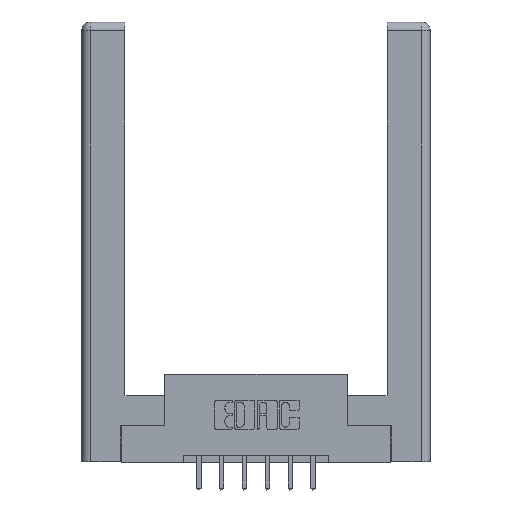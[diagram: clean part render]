
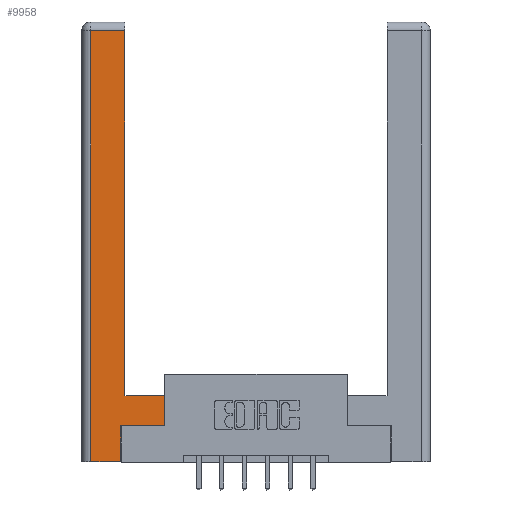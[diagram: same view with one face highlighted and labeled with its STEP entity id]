
A CAD part, top view. The second image highlights one B-rep face of the part: STEP entity #9958.
In plain terms, the highlighted planar face has unit normal (0, 0, 1).
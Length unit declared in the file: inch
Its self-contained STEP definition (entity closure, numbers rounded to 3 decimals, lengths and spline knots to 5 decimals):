
#147 = DIRECTION ( 'NONE',  ( -1., 0., 0. ) ) ;
#151 = ORIENTED_EDGE ( 'NONE', *, *, #1602, .T. ) ;
#175 = DIRECTION ( 'NONE',  ( 0., 1., 0. ) ) ;
#335 = CARTESIAN_POINT ( 'NONE',  ( 0.295, 0.45, 0. ) ) ;
#635 = CARTESIAN_POINT ( 'NONE',  ( 0.295, 2.94, 0. ) ) ;
#1460 = VECTOR ( 'NONE', #175, 39.37008 ) ;
#1470 = CARTESIAN_POINT ( 'NONE',  ( 0.565, 0.45, 0. ) ) ;
#1513 = CARTESIAN_POINT ( 'NONE',  ( 0.0615, 0., 0. ) ) ;
#1544 = VECTOR ( 'NONE', #8016, 39.37008 ) ;
#1602 = EDGE_CURVE ( 'NONE', #4958, #4509, #4754, .T. ) ;
#1690 = ORIENTED_EDGE ( 'NONE', *, *, #8846, .T. ) ;
#1697 = VECTOR ( 'NONE', #11351, 39.37008 ) ;
#1726 = LINE ( 'NONE', #1470, #5776 ) ;
#1737 = EDGE_CURVE ( 'NONE', #10759, #4958, #9622, .T. ) ;
#2299 = VECTOR ( 'NONE', #7509, 39.37008 ) ;
#2758 = VERTEX_POINT ( 'NONE', #9041 ) ;
#2831 = VECTOR ( 'NONE', #10468, 39.37008 ) ;
#3073 = VERTEX_POINT ( 'NONE', #9050 ) ;
#3211 = EDGE_LOOP ( 'NONE', ( #3826, #151, #6633, #1690, #8529, #4054, #4448, #8584 ) ) ;
#3506 = DIRECTION ( 'NONE',  ( 0., 1., 0. ) ) ;
#3643 = CARTESIAN_POINT ( 'NONE',  ( 0.0615, 0., 0. ) ) ;
#3826 = ORIENTED_EDGE ( 'NONE', *, *, #1737, .T. ) ;
#3827 = CARTESIAN_POINT ( 'NONE',  ( 0.0615, 2.94, 0. ) ) ;
#4054 = ORIENTED_EDGE ( 'NONE', *, *, #5088, .T. ) ;
#4255 = EDGE_CURVE ( 'NONE', #9108, #3073, #1726, .T. ) ;
#4448 = ORIENTED_EDGE ( 'NONE', *, *, #4255, .T. ) ;
#4509 = VERTEX_POINT ( 'NONE', #4543 ) ;
#4543 = CARTESIAN_POINT ( 'NONE',  ( 0.0615, 2.94, 0. ) ) ;
#4549 = CARTESIAN_POINT ( 'NONE',  ( 0.265, 0.245, 0. ) ) ;
#4693 = DIRECTION ( 'NONE',  ( 0., 0., -1. ) ) ;
#4754 = LINE ( 'NONE', #3827, #2299 ) ;
#4848 = FACE_OUTER_BOUND ( 'NONE', #3211, .T. ) ;
#4958 = VERTEX_POINT ( 'NONE', #635 ) ;
#5088 = EDGE_CURVE ( 'NONE', #5281, #9108, #8561, .T. ) ;
#5151 = VECTOR ( 'NONE', #8184, 39.37008 ) ;
#5281 = VERTEX_POINT ( 'NONE', #7775 ) ;
#5704 = CARTESIAN_POINT ( 'NONE',  ( 0., 0., 0. ) ) ;
#5728 = CARTESIAN_POINT ( 'NONE',  ( 0.295, 3., 0. ) ) ;
#5776 = VECTOR ( 'NONE', #3506, 39.37008 ) ;
#6212 = VECTOR ( 'NONE', #11105, 39.37008 ) ;
#6410 = CARTESIAN_POINT ( 'NONE',  ( 0.565, 0.245, 0. ) ) ;
#6633 = ORIENTED_EDGE ( 'NONE', *, *, #6708, .T. ) ;
#6708 = EDGE_CURVE ( 'NONE', #4509, #8497, #6783, .T. ) ;
#6783 = LINE ( 'NONE', #1513, #1544 ) ;
#6902 = LINE ( 'NONE', #335, #2831 ) ;
#7509 = DIRECTION ( 'NONE',  ( -1., 0., 0. ) ) ;
#7775 = CARTESIAN_POINT ( 'NONE',  ( 0.265, 0.245, 0. ) ) ;
#7872 = EDGE_CURVE ( 'NONE', #3073, #10759, #6902, .T. ) ;
#8016 = DIRECTION ( 'NONE',  ( 0., -1., 0. ) ) ;
#8184 = DIRECTION ( 'NONE',  ( 0., 1., 0. ) ) ;
#8497 = VERTEX_POINT ( 'NONE', #3643 ) ;
#8511 = CARTESIAN_POINT ( 'NONE',  ( 0.265, 0., 0. ) ) ;
#8529 = ORIENTED_EDGE ( 'NONE', *, *, #9444, .T. ) ;
#8561 = LINE ( 'NONE', #6410, #6212 ) ;
#8584 = ORIENTED_EDGE ( 'NONE', *, *, #7872, .T. ) ;
#8846 = EDGE_CURVE ( 'NONE', #8497, #2758, #12041, .T. ) ;
#9041 = CARTESIAN_POINT ( 'NONE',  ( 0.265, 0., 0. ) ) ;
#9050 = CARTESIAN_POINT ( 'NONE',  ( 0.565, 0.45, 0. ) ) ;
#9108 = VERTEX_POINT ( 'NONE', #9927 ) ;
#9444 = EDGE_CURVE ( 'NONE', #2758, #5281, #10391, .T. ) ;
#9622 = LINE ( 'NONE', #5728, #1460 ) ;
#9725 = CARTESIAN_POINT ( 'NONE',  ( 0.295, 0.45, 0. ) ) ;
#9927 = CARTESIAN_POINT ( 'NONE',  ( 0.565, 0.245, 0. ) ) ;
#9958 = ADVANCED_FACE ( 'NONE', ( #4848 ), #11304, .F. ) ;
#10391 = LINE ( 'NONE', #4549, #5151 ) ;
#10468 = DIRECTION ( 'NONE',  ( -1., 0., 0. ) ) ;
#10759 = VERTEX_POINT ( 'NONE', #9725 ) ;
#11057 = AXIS2_PLACEMENT_3D ( 'NONE', #5704, #4693, #147 ) ;
#11105 = DIRECTION ( 'NONE',  ( 1., 0., 0. ) ) ;
#11304 = PLANE ( 'NONE',  #11057 ) ;
#11351 = DIRECTION ( 'NONE',  ( 1., 0., 0. ) ) ;
#12041 = LINE ( 'NONE', #8511, #1697 ) ;
